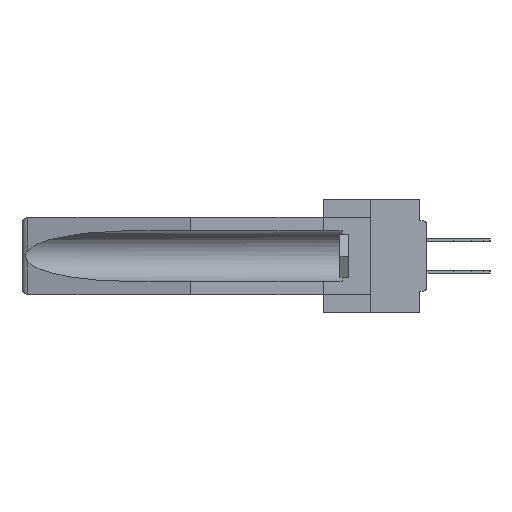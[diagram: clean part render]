
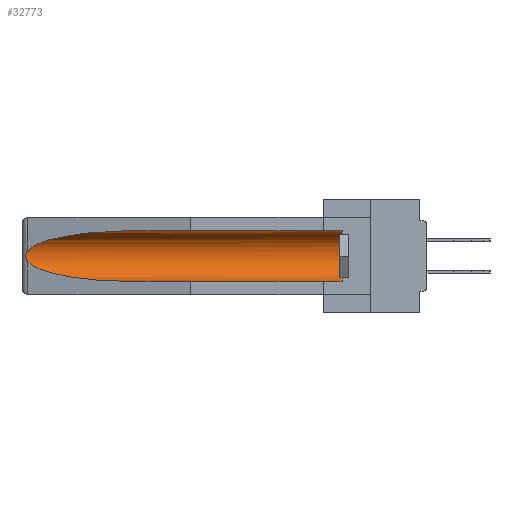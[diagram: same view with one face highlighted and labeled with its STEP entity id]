
A CAD part, left-side view. The second image highlights one B-rep face of the part: STEP entity #32773.
In plain terms, the highlighted cylindrical face has radius 2.857 mm (diameter 5.715 mm), a partial arc.
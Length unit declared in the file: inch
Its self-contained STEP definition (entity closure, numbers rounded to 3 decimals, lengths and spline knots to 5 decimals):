
#314 = EDGE_CURVE ( 'NONE', #11766, #17930, #7699, .T. ) ;
#367 = VERTEX_POINT ( 'NONE', #19606 ) ;
#497 = EDGE_LOOP ( 'NONE', ( #35315, #5518, #5046, #29904, #20352, #12082 ) ) ;
#866 = CARTESIAN_POINT ( 'NONE',  ( 0.21114, 1.30732, -0.059 ) ) ;
#1018 = FACE_OUTER_BOUND ( 'NONE', #497, .T. ) ;
#1459 = VECTOR ( 'NONE', #25223, 39.37008 ) ;
#1903 =( BOUNDED_CURVE ( )  B_SPLINE_CURVE ( 3, ( #16448, #8631, #33341, #21989 ),
 .UNSPECIFIED., .F., .T. ) 
 B_SPLINE_CURVE_WITH_KNOTS ( ( 4, 4 ),
 ( 0.1948, 1.5708 ),
 .UNSPECIFIED. ) 
 CURVE ( )  GEOMETRIC_REPRESENTATION_ITEM ( )  RATIONAL_B_SPLINE_CURVE ( ( 1., 0.848, 0.848, 1. ) ) 
 REPRESENTATION_ITEM ( '' )  );
#1999 = CIRCLE ( 'NONE', #14577, 0.1125 ) ;
#2479 = DIRECTION ( 'NONE',  ( 0., 0., 1. ) ) ;
#2585 = CARTESIAN_POINT ( 'NONE',  ( 0.155, 0.126, -0.059 ) ) ;
#2605 = CARTESIAN_POINT ( 'NONE',  ( 0.26597, 1.5296, -0.19026 ) ) ;
#2957 = CARTESIAN_POINT ( 'NONE',  ( 0.26655, 1.53094, -0.18657 ) ) ;
#3122 = CARTESIAN_POINT ( 'NONE',  ( 0.155, 1.07973, -0.059 ) ) ;
#3693 = EDGE_CURVE ( 'NONE', #367, #28327, #1903, .T. ) ;
#3699 = CARTESIAN_POINT ( 'NONE',  ( 0.155, -0.30754, -0.059 ) ) ;
#4197 = VERTEX_POINT ( 'NONE', #4842 ) ;
#4802 = EDGE_CURVE ( 'NONE', #26033, #367, #34819, .T. ) ;
#4842 = CARTESIAN_POINT ( 'NONE',  ( 0.155, 0.126, -0.284 ) ) ;
#5046 = ORIENTED_EDGE ( 'NONE', *, *, #3693, .T. ) ;
#5518 = ORIENTED_EDGE ( 'NONE', *, *, #4802, .T. ) ;
#5719 = CARTESIAN_POINT ( 'NONE',  ( 0.2673, 1.53269, -0.17917 ) ) ;
#5741 = CARTESIAN_POINT ( 'NONE',  ( 0.155, 1.07973, -0.059 ) ) ;
#5895 = CARTESIAN_POINT ( 'NONE',  ( 0.25451, 1.48313, -0.09465 ) ) ;
#6471 = DIRECTION ( 'NONE',  ( 0., 1., 0. ) ) ;
#7699 = LINE ( 'NONE', #3699, #32941 ) ;
#8377 = CARTESIAN_POINT ( 'NONE',  ( 0.26537, 1.52718, -0.19328 ) ) ;
#8631 = CARTESIAN_POINT ( 'NONE',  ( 0.25451, 1.48313, -0.24835 ) ) ;
#9533 = AXIS2_PLACEMENT_3D ( 'NONE', #29737, #11768, #2479 ) ;
#10837 = CARTESIAN_POINT ( 'NONE',  ( 0.2675, 1.53308, -0.16763 ) ) ;
#11766 = VERTEX_POINT ( 'NONE', #2585 ) ;
#11768 = DIRECTION ( 'NONE',  ( 0., 1., 0. ) ) ;
#12082 = ORIENTED_EDGE ( 'NONE', *, *, #314, .T. ) ;
#12897 = DIRECTION ( 'NONE',  ( 0., -1., 0. ) ) ;
#13127 = CARTESIAN_POINT ( 'NONE',  ( 0.155, 0.126, -0.1715 ) ) ;
#13257 = EDGE_CURVE ( 'NONE', #17930, #26033, #21641, .T. ) ;
#13699 = CARTESIAN_POINT ( 'NONE',  ( 0.26597, 1.52961, -0.15275 ) ) ;
#14577 = AXIS2_PLACEMENT_3D ( 'NONE', #13127, #12897, #26772 ) ;
#16148 = EDGE_CURVE ( 'NONE', #4197, #11766, #1999, .T. ) ;
#16442 = CARTESIAN_POINT ( 'NONE',  ( 0.2675, 1.53308, -0.17534 ) ) ;
#16448 = CARTESIAN_POINT ( 'NONE',  ( 0.26537, 1.52718, -0.19328 ) ) ;
#17268 = CYLINDRICAL_SURFACE ( 'NONE', #9533, 0.1125 ) ;
#17930 = VERTEX_POINT ( 'NONE', #5741 ) ;
#18976 = CARTESIAN_POINT ( 'NONE',  ( 0.26654, 1.53092, -0.15636 ) ) ;
#19606 = CARTESIAN_POINT ( 'NONE',  ( 0.26537, 1.52718, -0.19328 ) ) ;
#19853 = LINE ( 'NONE', #22271, #1459 ) ;
#20352 = ORIENTED_EDGE ( 'NONE', *, *, #16148, .T. ) ;
#21641 =( BOUNDED_CURVE ( )  B_SPLINE_CURVE ( 3, ( #3122, #866, #5895, #33158 ),
 .UNSPECIFIED., .F., .T. ) 
 B_SPLINE_CURVE_WITH_KNOTS ( ( 4, 4 ),
 ( 4.71239, 6.08839 ),
 .UNSPECIFIED. ) 
 CURVE ( )  GEOMETRIC_REPRESENTATION_ITEM ( )  RATIONAL_B_SPLINE_CURVE ( ( 1., 0.848, 0.848, 1. ) ) 
 REPRESENTATION_ITEM ( '' )  );
#21989 = CARTESIAN_POINT ( 'NONE',  ( 0.155, 1.07973, -0.284 ) ) ;
#22271 = CARTESIAN_POINT ( 'NONE',  ( 0.155, -0.30754, -0.284 ) ) ;
#22983 = CARTESIAN_POINT ( 'NONE',  ( 0.155, 1.07973, -0.284 ) ) ;
#23288 = CARTESIAN_POINT ( 'NONE',  ( 0.26537, 1.52718, -0.14972 ) ) ;
#25223 = DIRECTION ( 'NONE',  ( 0., 1., 0. ) ) ;
#26033 = VERTEX_POINT ( 'NONE', #23288 ) ;
#26772 = DIRECTION ( 'NONE',  ( 0., 0., 1. ) ) ;
#27337 = CARTESIAN_POINT ( 'NONE',  ( 0.26537, 1.52718, -0.14972 ) ) ;
#28327 = VERTEX_POINT ( 'NONE', #22983 ) ;
#29737 = CARTESIAN_POINT ( 'NONE',  ( 0.155, -0.30754, -0.1715 ) ) ;
#29904 = ORIENTED_EDGE ( 'NONE', *, *, #32302, .F. ) ;
#32302 = EDGE_CURVE ( 'NONE', #4197, #28327, #19853, .T. ) ;
#32755 = CARTESIAN_POINT ( 'NONE',  ( 0.2673, 1.5327, -0.16383 ) ) ;
#32773 = ADVANCED_FACE ( 'NONE', ( #1018 ), #17268, .F. ) ;
#32941 = VECTOR ( 'NONE', #6471, 39.37008 ) ;
#33158 = CARTESIAN_POINT ( 'NONE',  ( 0.26537, 1.52718, -0.14972 ) ) ;
#33341 = CARTESIAN_POINT ( 'NONE',  ( 0.21114, 1.30732, -0.284 ) ) ;
#34819 = B_SPLINE_CURVE_WITH_KNOTS ( 'NONE', 3,
 ( #27337, #13699, #18976, #32755, #10837, #16442, #5719, #2957, #2605, #8377 ),
 .UNSPECIFIED., .F., .F.,
 ( 4, 2, 2, 2, 4 ),
 ( 0., 0.00029, 0.00058, 0.00087, 0.00117 ),
 .UNSPECIFIED. ) ;
#35315 = ORIENTED_EDGE ( 'NONE', *, *, #13257, .T. ) ;
